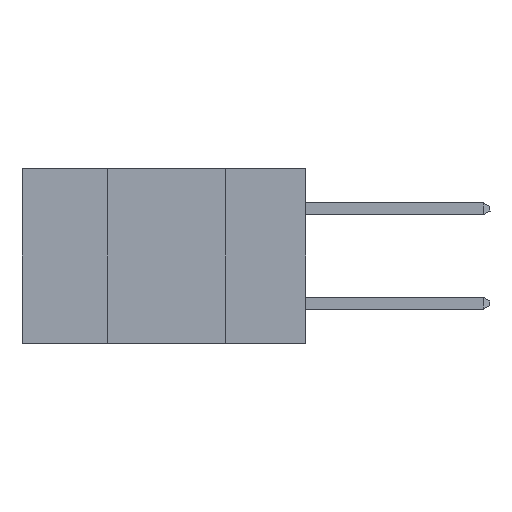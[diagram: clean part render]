
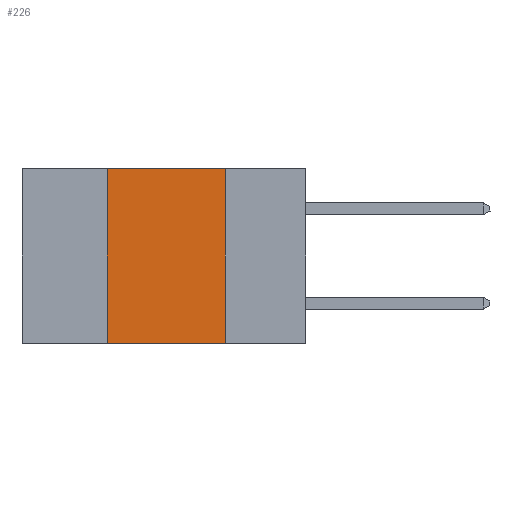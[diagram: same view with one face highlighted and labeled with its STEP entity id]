
A CAD part, left-side view. The second image highlights one B-rep face of the part: STEP entity #226.
In plain terms, the highlighted planar face has unit normal (-1, 0, 0).
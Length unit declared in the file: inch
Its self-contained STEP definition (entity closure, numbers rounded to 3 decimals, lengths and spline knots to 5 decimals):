
#226 = ADVANCED_FACE ( 'NONE', ( #16778 ), #9095, .F. ) ;
#375 = CARTESIAN_POINT ( 'NONE',  ( 0., 0.6, -0.37 ) ) ;
#2620 = ORIENTED_EDGE ( 'NONE', *, *, #25887, .F. ) ;
#5775 = DIRECTION ( 'NONE',  ( 0., -1., 0. ) ) ;
#6494 = VECTOR ( 'NONE', #5775, 39.37008 ) ;
#8589 = LINE ( 'NONE', #9522, #17069 ) ;
#9095 = PLANE ( 'NONE',  #19442 ) ;
#9522 = CARTESIAN_POINT ( 'NONE',  ( 0., 0.42, 0. ) ) ;
#9798 = EDGE_CURVE ( 'NONE', #27081, #12142, #15395, .T. ) ;
#10235 = CARTESIAN_POINT ( 'NONE',  ( 0., 0.17, 0. ) ) ;
#12142 = VERTEX_POINT ( 'NONE', #10235 ) ;
#12713 = VECTOR ( 'NONE', #25264, 39.37008 ) ;
#12843 = ORIENTED_EDGE ( 'NONE', *, *, #27791, .T. ) ;
#13234 = CARTESIAN_POINT ( 'NONE',  ( 0., 0.6, 0. ) ) ;
#15299 = ORIENTED_EDGE ( 'NONE', *, *, #23221, .F. ) ;
#15395 = LINE ( 'NONE', #13234, #19619 ) ;
#16778 = FACE_OUTER_BOUND ( 'NONE', #31420, .T. ) ;
#17069 = VECTOR ( 'NONE', #31506, 39.37008 ) ;
#19240 = LINE ( 'NONE', #22771, #12713 ) ;
#19442 = AXIS2_PLACEMENT_3D ( 'NONE', #26362, #28825, #28613 ) ;
#19619 = VECTOR ( 'NONE', #28193, 39.37008 ) ;
#21531 = LINE ( 'NONE', #375, #6494 ) ;
#22771 = CARTESIAN_POINT ( 'NONE',  ( 0., 0.17, 0. ) ) ;
#23221 = EDGE_CURVE ( 'NONE', #12142, #28506, #19240, .T. ) ;
#23480 = CARTESIAN_POINT ( 'NONE',  ( 0., 0.42, -0.37 ) ) ;
#25264 = DIRECTION ( 'NONE',  ( 0., 0., -1. ) ) ;
#25887 = EDGE_CURVE ( 'NONE', #29915, #27081, #8589, .T. ) ;
#26362 = CARTESIAN_POINT ( 'NONE',  ( 0., 0.6, 0. ) ) ;
#27081 = VERTEX_POINT ( 'NONE', #28951 ) ;
#27791 = EDGE_CURVE ( 'NONE', #29915, #28506, #21531, .T. ) ;
#28193 = DIRECTION ( 'NONE',  ( 0., -1., 0. ) ) ;
#28506 = VERTEX_POINT ( 'NONE', #29535 ) ;
#28613 = DIRECTION ( 'NONE',  ( 0., 0., -1. ) ) ;
#28825 = DIRECTION ( 'NONE',  ( 1., 0., 0. ) ) ;
#28951 = CARTESIAN_POINT ( 'NONE',  ( 0., 0.42, 0. ) ) ;
#29185 = ORIENTED_EDGE ( 'NONE', *, *, #9798, .F. ) ;
#29535 = CARTESIAN_POINT ( 'NONE',  ( 0., 0.17, -0.37 ) ) ;
#29915 = VERTEX_POINT ( 'NONE', #23480 ) ;
#31420 = EDGE_LOOP ( 'NONE', ( #15299, #29185, #2620, #12843 ) ) ;
#31506 = DIRECTION ( 'NONE',  ( 0., 0., 1. ) ) ;
